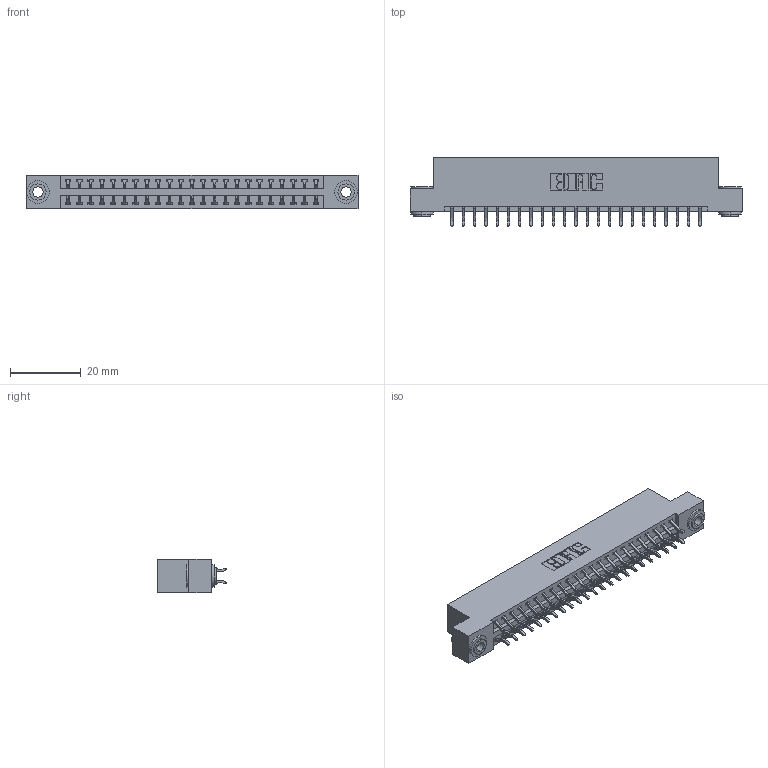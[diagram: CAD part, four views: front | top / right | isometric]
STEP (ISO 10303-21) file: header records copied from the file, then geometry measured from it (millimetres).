
FILE_DESCRIPTION (( 'STEP AP203' ), '1' );
FILE_NAME ('396-046-556-203.STEP', '2019-10-30T12:10:25', ( '' ), ( '' ), 'SwSTEP 2.0', 'SolidWorks 2016', '' );
FILE_SCHEMA (( 'CONFIG_CONTROL_DESIGN' ));
Length unit declared in the file: inch
Products named in the file (4): 396-046-556-203; 345-292-001_556 Tail; 345-250-002_345-250-002-102; 346 Part_Flush Mounting Lugs - 0.156 Dia-TH
Assembly tree (49 placements, depth 2):
  396-046-556-203
    346 Part_Flush Mounting Lugs - 0.156 Dia-TH
    345-292-001_556 Tail  x46
    345-250-002_345-250-002-102  x2
Bounding box: 93.6 x 19.57 x 9.4 mm (x, y, z)
Volume: 8997.1 mm3; surface area: 12239.9 mm2
Topology: 49 solids, 49 shells, 2828 faces, 8363 edges, 5510 vertices
Faces by surface type: plane 1880, cylinder 940, cone 8
Entity records: 18438 total; most frequent: CARTESIAN_POINT 3055, ORIENTED_EDGE 2970, DIRECTION 2763, EDGE_CURVE 1485, VECTOR 1229, LINE 1229, VERTEX_POINT 986, AXIS2_PLACEMENT_3D 767
